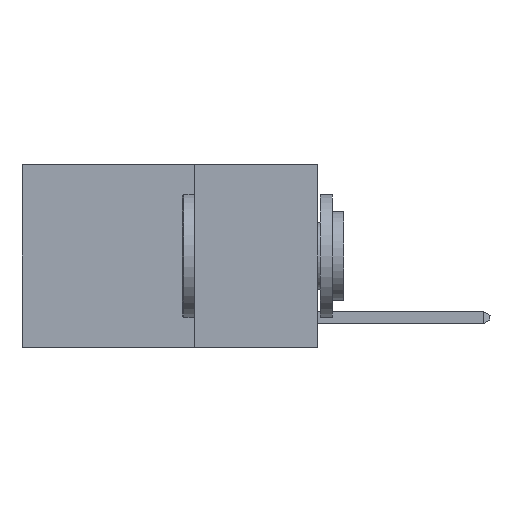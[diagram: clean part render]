
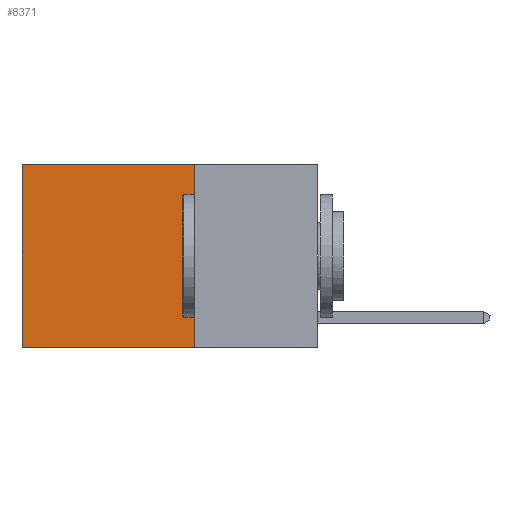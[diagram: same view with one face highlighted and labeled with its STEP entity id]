
A CAD part, left-side view. The second image highlights one B-rep face of the part: STEP entity #8371.
In plain terms, the highlighted planar face has unit normal (-1, 0, 0).
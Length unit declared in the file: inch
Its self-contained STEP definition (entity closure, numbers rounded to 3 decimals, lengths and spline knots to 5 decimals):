
#882 = VECTOR ( 'NONE', #1831, 39.37008 ) ;
#1375 = LINE ( 'NONE', #20720, #17760 ) ;
#1536 = VECTOR ( 'NONE', #8425, 39.37008 ) ;
#1831 = DIRECTION ( 'NONE',  ( 0., 1., 0. ) ) ;
#2395 = ORIENTED_EDGE ( 'NONE', *, *, #19345, .F. ) ;
#2754 = AXIS2_PLACEMENT_3D ( 'NONE', #4975, #20847, #20738 ) ;
#3371 = VERTEX_POINT ( 'NONE', #8741 ) ;
#4975 = CARTESIAN_POINT ( 'NONE',  ( 0.2625, 0.25, 0. ) ) ;
#5061 = EDGE_CURVE ( 'NONE', #3371, #12971, #10699, .T. ) ;
#6009 = DIRECTION ( 'NONE',  ( 0., 0., -1. ) ) ;
#6661 = CARTESIAN_POINT ( 'NONE',  ( 0.2625, 0.25, -0.37 ) ) ;
#7675 = VECTOR ( 'NONE', #6009, 39.37008 ) ;
#7728 = ORIENTED_EDGE ( 'NONE', *, *, #5061, .T. ) ;
#7743 = CARTESIAN_POINT ( 'NONE',  ( 0.2625, 0.6, -0.37 ) ) ;
#8224 = CARTESIAN_POINT ( 'NONE',  ( 0.2625, 0.25, 0. ) ) ;
#8371 = ADVANCED_FACE ( 'NONE', ( #15463 ), #17081, .F. ) ;
#8377 = DIRECTION ( 'NONE',  ( 0., 1., 0. ) ) ;
#8425 = DIRECTION ( 'NONE',  ( 0., 0., -1. ) ) ;
#8534 = LINE ( 'NONE', #8224, #1536 ) ;
#8741 = CARTESIAN_POINT ( 'NONE',  ( 0.2625, 0.25, 0. ) ) ;
#9050 = CARTESIAN_POINT ( 'NONE',  ( 0.2625, 0.6, 0. ) ) ;
#9934 = ORIENTED_EDGE ( 'NONE', *, *, #19748, .F. ) ;
#10699 = LINE ( 'NONE', #17770, #882 ) ;
#12022 = EDGE_LOOP ( 'NONE', ( #15207, #9934, #2395, #7728 ) ) ;
#12934 = CARTESIAN_POINT ( 'NONE',  ( 0.2625, 0.6, 0. ) ) ;
#12971 = VERTEX_POINT ( 'NONE', #12934 ) ;
#14637 = EDGE_CURVE ( 'NONE', #12971, #20226, #21773, .T. ) ;
#15207 = ORIENTED_EDGE ( 'NONE', *, *, #14637, .T. ) ;
#15463 = FACE_OUTER_BOUND ( 'NONE', #12022, .T. ) ;
#17081 = PLANE ( 'NONE',  #2754 ) ;
#17760 = VECTOR ( 'NONE', #8377, 39.37008 ) ;
#17770 = CARTESIAN_POINT ( 'NONE',  ( 0.2625, 0.25, 0. ) ) ;
#19345 = EDGE_CURVE ( 'NONE', #3371, #19764, #8534, .T. ) ;
#19748 = EDGE_CURVE ( 'NONE', #19764, #20226, #1375, .T. ) ;
#19764 = VERTEX_POINT ( 'NONE', #6661 ) ;
#20226 = VERTEX_POINT ( 'NONE', #7743 ) ;
#20720 = CARTESIAN_POINT ( 'NONE',  ( 0.2625, 0.25, -0.37 ) ) ;
#20738 = DIRECTION ( 'NONE',  ( 0., 0., -1. ) ) ;
#20847 = DIRECTION ( 'NONE',  ( 1., 0., 0. ) ) ;
#21773 = LINE ( 'NONE', #9050, #7675 ) ;
